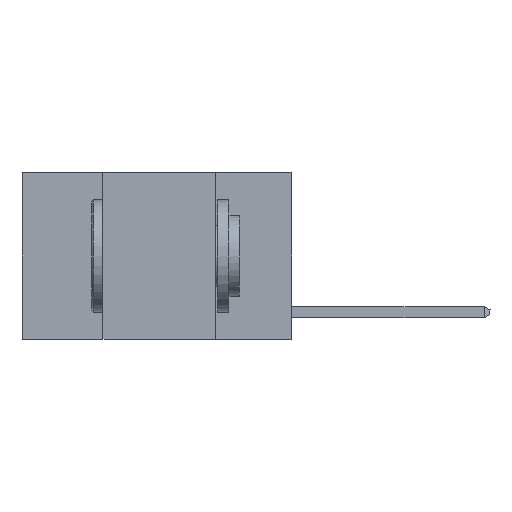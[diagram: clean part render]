
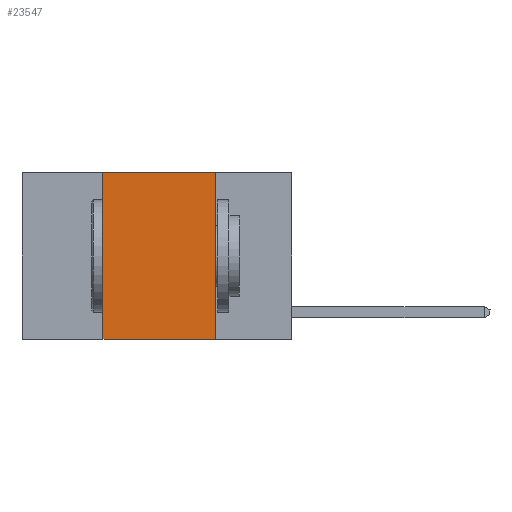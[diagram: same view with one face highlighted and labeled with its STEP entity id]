
A CAD part, left-side view. The second image highlights one B-rep face of the part: STEP entity #23547.
In plain terms, the highlighted planar face has unit normal (-1, 0, 0).
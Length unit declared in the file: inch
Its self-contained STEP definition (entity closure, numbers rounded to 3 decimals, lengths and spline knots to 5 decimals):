
#644 = CARTESIAN_POINT ( 'NONE',  ( 0., 0.17, 0. ) ) ;
#762 = VECTOR ( 'NONE', #9007, 39.37008 ) ;
#1206 = CARTESIAN_POINT ( 'NONE',  ( 0., 0.17, -0.37 ) ) ;
#3167 = ORIENTED_EDGE ( 'NONE', *, *, #4683, .T. ) ;
#3922 = EDGE_LOOP ( 'NONE', ( #24797, #18021, #24984, #3167 ) ) ;
#4047 = EDGE_CURVE ( 'NONE', #6853, #7318, #12322, .T. ) ;
#4683 = EDGE_CURVE ( 'NONE', #23162, #23061, #16909, .T. ) ;
#6853 = VERTEX_POINT ( 'NONE', #12021 ) ;
#7318 = VERTEX_POINT ( 'NONE', #644 ) ;
#8001 = AXIS2_PLACEMENT_3D ( 'NONE', #19763, #24042, #11384 ) ;
#8567 = CARTESIAN_POINT ( 'NONE',  ( 0., 0.17, 0. ) ) ;
#9007 = DIRECTION ( 'NONE',  ( 0., 0., 1. ) ) ;
#11318 = VECTOR ( 'NONE', #13234, 39.37008 ) ;
#11384 = DIRECTION ( 'NONE',  ( 0., 0., -1. ) ) ;
#11804 = FACE_OUTER_BOUND ( 'NONE', #3922, .T. ) ;
#12021 = CARTESIAN_POINT ( 'NONE',  ( 0., 0.42, 0. ) ) ;
#12120 = CARTESIAN_POINT ( 'NONE',  ( 0., 0.42, -0.37 ) ) ;
#12322 = LINE ( 'NONE', #25438, #17269 ) ;
#12788 = DIRECTION ( 'NONE',  ( 0., -1., 0. ) ) ;
#13234 = DIRECTION ( 'NONE',  ( 0., -1., 0. ) ) ;
#14909 = DIRECTION ( 'NONE',  ( 0., 0., -1. ) ) ;
#16909 = LINE ( 'NONE', #21653, #11318 ) ;
#17269 = VECTOR ( 'NONE', #12788, 39.37008 ) ;
#17539 = PLANE ( 'NONE',  #8001 ) ;
#18021 = ORIENTED_EDGE ( 'NONE', *, *, #4047, .F. ) ;
#18825 = EDGE_CURVE ( 'NONE', #23162, #6853, #23276, .T. ) ;
#19763 = CARTESIAN_POINT ( 'NONE',  ( 0., 0.6, 0. ) ) ;
#21653 = CARTESIAN_POINT ( 'NONE',  ( 0., 0.6, -0.37 ) ) ;
#23061 = VERTEX_POINT ( 'NONE', #1206 ) ;
#23162 = VERTEX_POINT ( 'NONE', #12120 ) ;
#23276 = LINE ( 'NONE', #23811, #762 ) ;
#23547 = ADVANCED_FACE ( 'NONE', ( #11804 ), #17539, .F. ) ;
#23811 = CARTESIAN_POINT ( 'NONE',  ( 0., 0.42, 0. ) ) ;
#24042 = DIRECTION ( 'NONE',  ( 1., 0., 0. ) ) ;
#24797 = ORIENTED_EDGE ( 'NONE', *, *, #25932, .F. ) ;
#24946 = VECTOR ( 'NONE', #14909, 39.37008 ) ;
#24984 = ORIENTED_EDGE ( 'NONE', *, *, #18825, .F. ) ;
#25438 = CARTESIAN_POINT ( 'NONE',  ( 0., 0.6, 0. ) ) ;
#25601 = LINE ( 'NONE', #8567, #24946 ) ;
#25932 = EDGE_CURVE ( 'NONE', #7318, #23061, #25601, .T. ) ;
